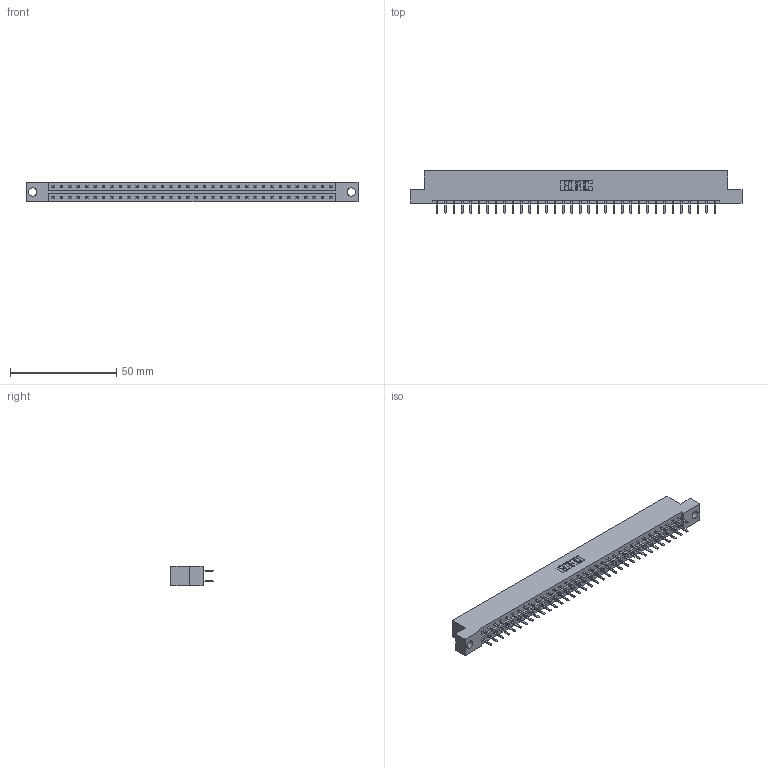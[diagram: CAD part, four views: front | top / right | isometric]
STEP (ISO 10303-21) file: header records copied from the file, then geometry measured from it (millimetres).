
FILE_DESCRIPTION (( 'STEP AP203' ), '1' );
FILE_NAME ('333-068-520-204.STEP', '2018-08-04T12:28:18', ( '' ), ( '' ), 'SwSTEP 2.0', 'SolidWorks 2016', '' );
FILE_SCHEMA (( 'CONFIG_CONTROL_DESIGN' ));
Length unit declared in the file: inch
Products named in the file (3): 333 Part_Flush - .156 Dia - TH; 345-292-001_345-293-120; 333-068-520-204
Assembly tree (69 placements, depth 2):
  333-068-520-204
    333 Part_Flush - .156 Dia - TH
    345-292-001_345-293-120  x68
Bounding box: 156.26 x 20.02 x 9.4 mm (x, y, z)
Volume: 15760.8 mm3; surface area: 18267.4 mm2
Topology: 69 solids, 69 shells, 3922 faces, 11395 edges, 7414 vertices
Faces by surface type: plane 2654, cylinder 1268
Entity records: 23025 total; most frequent: CARTESIAN_POINT 3838, ORIENTED_EDGE 3762, DIRECTION 3281, EDGE_CURVE 1881, LINE 1749, VECTOR 1749, VERTEX_POINT 1250, AXIS2_PLACEMENT_3D 766
